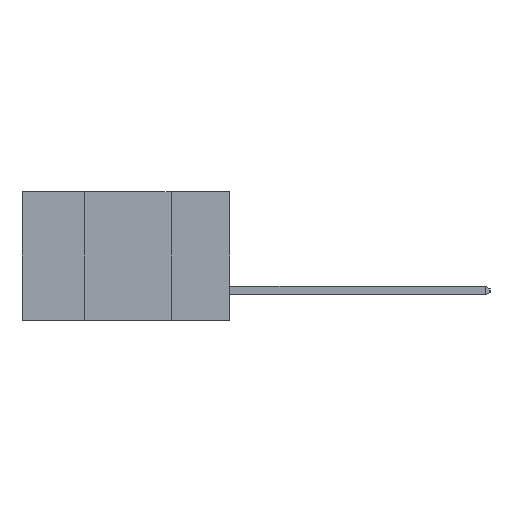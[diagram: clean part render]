
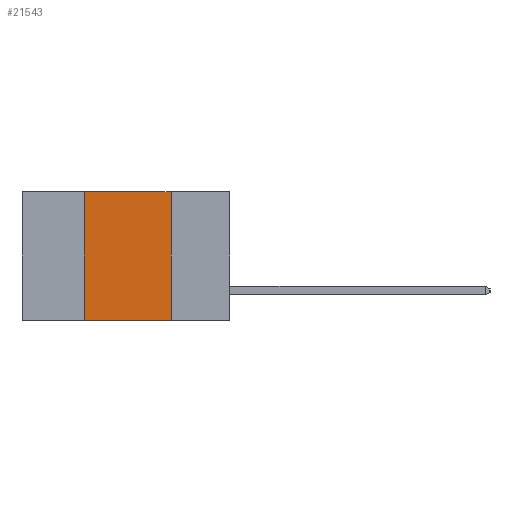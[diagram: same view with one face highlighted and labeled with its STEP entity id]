
A CAD part, left-side view. The second image highlights one B-rep face of the part: STEP entity #21543.
In plain terms, the highlighted planar face has unit normal (-1, 0, 0).
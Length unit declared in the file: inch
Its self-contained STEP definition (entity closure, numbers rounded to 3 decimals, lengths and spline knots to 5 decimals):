
#378 = DIRECTION ( 'NONE',  ( 0., 0., -1. ) ) ;
#1111 = ORIENTED_EDGE ( 'NONE', *, *, #16716, .T. ) ;
#3354 = EDGE_CURVE ( 'NONE', #16574, #16202, #14957, .T. ) ;
#4502 = ORIENTED_EDGE ( 'NONE', *, *, #17868, .F. ) ;
#5524 = VECTOR ( 'NONE', #19583, 39.37008 ) ;
#6011 = EDGE_LOOP ( 'NONE', ( #7851, #6221, #4502, #1111 ) ) ;
#6078 = CARTESIAN_POINT ( 'NONE',  ( 0., 0.6, -0.37 ) ) ;
#6221 = ORIENTED_EDGE ( 'NONE', *, *, #3354, .F. ) ;
#6518 = AXIS2_PLACEMENT_3D ( 'NONE', #19211, #22503, #12267 ) ;
#6699 = VECTOR ( 'NONE', #16866, 39.37008 ) ;
#7551 = LINE ( 'NONE', #6078, #20836 ) ;
#7660 = CARTESIAN_POINT ( 'NONE',  ( 0., 0.6, 0. ) ) ;
#7851 = ORIENTED_EDGE ( 'NONE', *, *, #21202, .F. ) ;
#10005 = VERTEX_POINT ( 'NONE', #10491 ) ;
#10205 = LINE ( 'NONE', #16137, #5524 ) ;
#10475 = PLANE ( 'NONE',  #6518 ) ;
#10491 = CARTESIAN_POINT ( 'NONE',  ( 0., 0.42, -0.37 ) ) ;
#11746 = CARTESIAN_POINT ( 'NONE',  ( 0., 0.17, -0.37 ) ) ;
#12267 = DIRECTION ( 'NONE',  ( 0., 0., -1. ) ) ;
#12754 = CARTESIAN_POINT ( 'NONE',  ( 0., 0.17, 0. ) ) ;
#13158 = DIRECTION ( 'NONE',  ( 0., -1., 0. ) ) ;
#14783 = FACE_OUTER_BOUND ( 'NONE', #6011, .T. ) ;
#14957 = LINE ( 'NONE', #7660, #6699 ) ;
#16137 = CARTESIAN_POINT ( 'NONE',  ( 0., 0.42, 0. ) ) ;
#16202 = VERTEX_POINT ( 'NONE', #21991 ) ;
#16574 = VERTEX_POINT ( 'NONE', #19695 ) ;
#16716 = EDGE_CURVE ( 'NONE', #10005, #20943, #7551, .T. ) ;
#16866 = DIRECTION ( 'NONE',  ( 0., -1., 0. ) ) ;
#17868 = EDGE_CURVE ( 'NONE', #10005, #16574, #10205, .T. ) ;
#18354 = VECTOR ( 'NONE', #378, 39.37008 ) ;
#19211 = CARTESIAN_POINT ( 'NONE',  ( 0., 0.6, 0. ) ) ;
#19412 = LINE ( 'NONE', #12754, #18354 ) ;
#19583 = DIRECTION ( 'NONE',  ( 0., 0., 1. ) ) ;
#19695 = CARTESIAN_POINT ( 'NONE',  ( 0., 0.42, 0. ) ) ;
#20836 = VECTOR ( 'NONE', #13158, 39.37008 ) ;
#20943 = VERTEX_POINT ( 'NONE', #11746 ) ;
#21202 = EDGE_CURVE ( 'NONE', #16202, #20943, #19412, .T. ) ;
#21543 = ADVANCED_FACE ( 'NONE', ( #14783 ), #10475, .F. ) ;
#21991 = CARTESIAN_POINT ( 'NONE',  ( 0., 0.17, 0. ) ) ;
#22503 = DIRECTION ( 'NONE',  ( 1., 0., 0. ) ) ;
